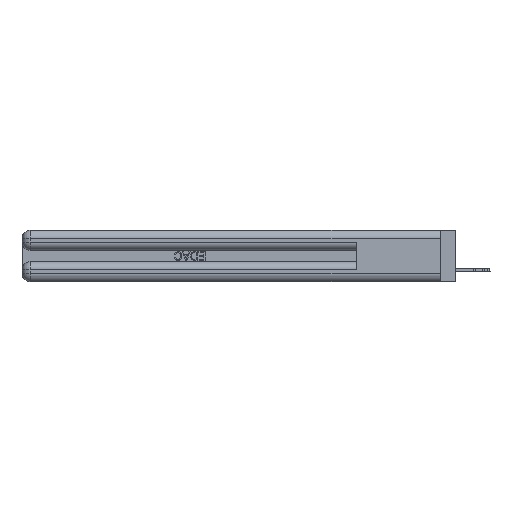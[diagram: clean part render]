
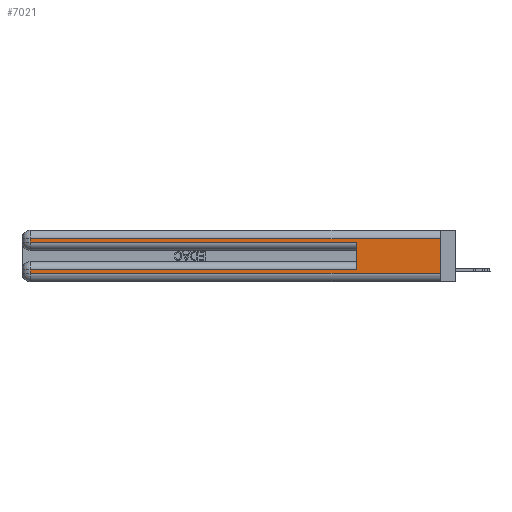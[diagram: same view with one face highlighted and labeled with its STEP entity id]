
A CAD part, left-side view. The second image highlights one B-rep face of the part: STEP entity #7021.
In plain terms, the highlighted planar face has unit normal (-1, 0, 0).
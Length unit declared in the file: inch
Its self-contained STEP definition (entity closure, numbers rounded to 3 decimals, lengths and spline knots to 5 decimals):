
#551 = LINE ( 'NONE', #37739, #26566 ) ;
#867 = LINE ( 'NONE', #33291, #18540 ) ;
#1419 = CARTESIAN_POINT ( 'NONE',  ( 0., 2.94, 0.37 ) ) ;
#1729 = ORIENTED_EDGE ( 'NONE', *, *, #15859, .T. ) ;
#1948 = VERTEX_POINT ( 'NONE', #21780 ) ;
#2816 = PLANE ( 'NONE',  #9786 ) ;
#3088 = LINE ( 'NONE', #21973, #10788 ) ;
#3292 = CARTESIAN_POINT ( 'NONE',  ( 0., 2.94, 0.285 ) ) ;
#3571 = VECTOR ( 'NONE', #14726, 39.37008 ) ;
#5649 = VERTEX_POINT ( 'NONE', #32551 ) ;
#6527 = LINE ( 'NONE', #29186, #17402 ) ;
#7021 = ADVANCED_FACE ( 'NONE', ( #42052 ), #2816, .F. ) ;
#7029 = EDGE_CURVE ( 'NONE', #8266, #32077, #10826, .T. ) ;
#8233 = CARTESIAN_POINT ( 'NONE',  ( 0., 2.94, 0.085 ) ) ;
#8266 = VERTEX_POINT ( 'NONE', #26161 ) ;
#9786 = AXIS2_PLACEMENT_3D ( 'NONE', #22673, #22375, #25725 ) ;
#9919 = DIRECTION ( 'NONE',  ( 0., 0., 1. ) ) ;
#10788 = VECTOR ( 'NONE', #31229, 39.37008 ) ;
#10826 = LINE ( 'NONE', #12326, #31074 ) ;
#11705 = CARTESIAN_POINT ( 'NONE',  ( 0., 0., 0.285 ) ) ;
#12326 = CARTESIAN_POINT ( 'NONE',  ( 0., 0., 0.37 ) ) ;
#14726 = DIRECTION ( 'NONE',  ( 0., 0., -1. ) ) ;
#14813 = DIRECTION ( 'NONE',  ( 0., 0., -1. ) ) ;
#15367 = DIRECTION ( 'NONE',  ( 0., -1., 0. ) ) ;
#15859 = EDGE_CURVE ( 'NONE', #23467, #26795, #30822, .T. ) ;
#16393 = DIRECTION ( 'NONE',  ( 0., 1., 0. ) ) ;
#17402 = VECTOR ( 'NONE', #16393, 39.37008 ) ;
#18114 = LINE ( 'NONE', #1419, #3571 ) ;
#18329 = ORIENTED_EDGE ( 'NONE', *, *, #33831, .T. ) ;
#18540 = VECTOR ( 'NONE', #9919, 39.37008 ) ;
#20402 = ORIENTED_EDGE ( 'NONE', *, *, #7029, .F. ) ;
#20600 = EDGE_CURVE ( 'NONE', #8266, #5649, #551, .T. ) ;
#21417 = CARTESIAN_POINT ( 'NONE',  ( 0., 0.6, 0.085 ) ) ;
#21780 = CARTESIAN_POINT ( 'NONE',  ( 0., 0.6, 0.285 ) ) ;
#21973 = CARTESIAN_POINT ( 'NONE',  ( 0., 0., 0.06 ) ) ;
#22375 = DIRECTION ( 'NONE',  ( 1., 0., 0. ) ) ;
#22632 = CARTESIAN_POINT ( 'NONE',  ( 0., 0., 0.06 ) ) ;
#22673 = CARTESIAN_POINT ( 'NONE',  ( 0., 0., 0.37 ) ) ;
#22846 = ORIENTED_EDGE ( 'NONE', *, *, #31855, .T. ) ;
#23467 = VERTEX_POINT ( 'NONE', #8233 ) ;
#24588 = VECTOR ( 'NONE', #14813, 39.37008 ) ;
#24598 = EDGE_CURVE ( 'NONE', #26795, #32077, #3088, .T. ) ;
#25204 = ORIENTED_EDGE ( 'NONE', *, *, #20600, .T. ) ;
#25725 = DIRECTION ( 'NONE',  ( 0., 0., -1. ) ) ;
#26147 = VERTEX_POINT ( 'NONE', #3292 ) ;
#26161 = CARTESIAN_POINT ( 'NONE',  ( 0., 0., 0.31 ) ) ;
#26275 = CARTESIAN_POINT ( 'NONE',  ( 0., 2.94, 0.06 ) ) ;
#26566 = VECTOR ( 'NONE', #36312, 39.37008 ) ;
#26795 = VERTEX_POINT ( 'NONE', #26275 ) ;
#29186 = CARTESIAN_POINT ( 'NONE',  ( 0., 0., 0.085 ) ) ;
#30822 = LINE ( 'NONE', #37459, #24588 ) ;
#31074 = VECTOR ( 'NONE', #38757, 39.37008 ) ;
#31228 = EDGE_CURVE ( 'NONE', #26147, #1948, #31639, .T. ) ;
#31229 = DIRECTION ( 'NONE',  ( 0., -1., 0. ) ) ;
#31639 = LINE ( 'NONE', #11705, #42641 ) ;
#31855 = EDGE_CURVE ( 'NONE', #5649, #26147, #18114, .T. ) ;
#32077 = VERTEX_POINT ( 'NONE', #22632 ) ;
#32551 = CARTESIAN_POINT ( 'NONE',  ( 0., 2.94, 0.31 ) ) ;
#32838 = EDGE_CURVE ( 'NONE', #36668, #1948, #867, .T. ) ;
#33291 = CARTESIAN_POINT ( 'NONE',  ( 0., 0.6, 0.145 ) ) ;
#33831 = EDGE_CURVE ( 'NONE', #36668, #23467, #6527, .T. ) ;
#34648 = ORIENTED_EDGE ( 'NONE', *, *, #24598, .T. ) ;
#36312 = DIRECTION ( 'NONE',  ( 0., 1., 0. ) ) ;
#36668 = VERTEX_POINT ( 'NONE', #21417 ) ;
#37155 = ORIENTED_EDGE ( 'NONE', *, *, #32838, .F. ) ;
#37411 = EDGE_LOOP ( 'NONE', ( #20402, #25204, #22846, #39678, #37155, #18329, #1729, #34648 ) ) ;
#37459 = CARTESIAN_POINT ( 'NONE',  ( 0., 2.94, 0.37 ) ) ;
#37739 = CARTESIAN_POINT ( 'NONE',  ( 0., 0., 0.31 ) ) ;
#38757 = DIRECTION ( 'NONE',  ( 0., 0., -1. ) ) ;
#39678 = ORIENTED_EDGE ( 'NONE', *, *, #31228, .T. ) ;
#42052 = FACE_OUTER_BOUND ( 'NONE', #37411, .T. ) ;
#42641 = VECTOR ( 'NONE', #15367, 39.37008 ) ;
